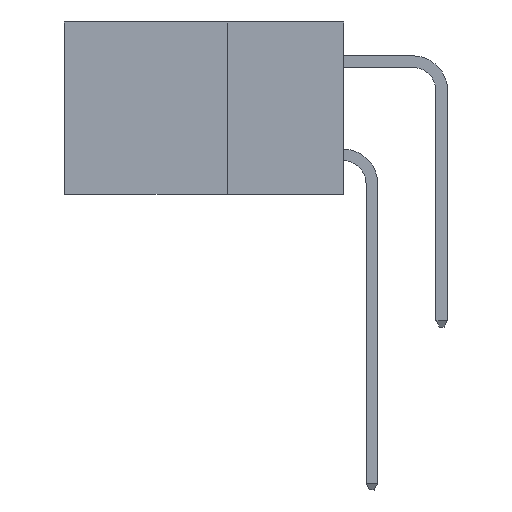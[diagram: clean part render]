
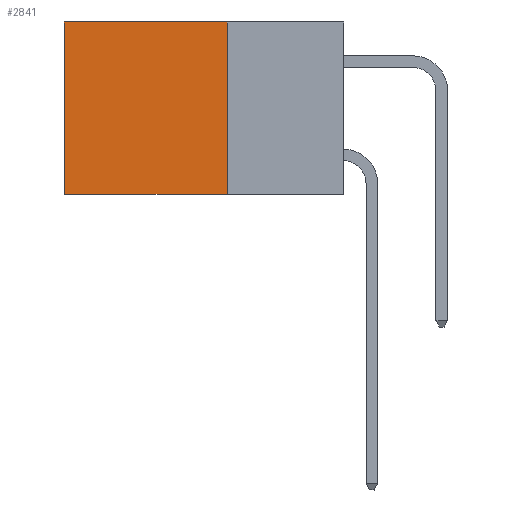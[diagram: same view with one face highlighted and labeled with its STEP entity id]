
A CAD part, left-side view. The second image highlights one B-rep face of the part: STEP entity #2841.
In plain terms, the highlighted planar face has unit normal (-1, 0, 0).
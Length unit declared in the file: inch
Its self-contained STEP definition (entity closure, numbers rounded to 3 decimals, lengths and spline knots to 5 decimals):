
#200 = CARTESIAN_POINT ( 'NONE',  ( 0.298, 0.25, -0.37 ) ) ;
#350 = EDGE_CURVE ( 'NONE', #2766, #12796, #1570, .T. ) ;
#964 = LINE ( 'NONE', #6120, #3939 ) ;
#1142 = VECTOR ( 'NONE', #9145, 39.37008 ) ;
#1369 = VECTOR ( 'NONE', #1447, 39.37008 ) ;
#1447 = DIRECTION ( 'NONE',  ( 0., 1., 0. ) ) ;
#1570 = LINE ( 'NONE', #13937, #1966 ) ;
#1756 = LINE ( 'NONE', #200, #1369 ) ;
#1966 = VECTOR ( 'NONE', #3776, 39.37008 ) ;
#2536 = DIRECTION ( 'NONE',  ( 0., 0., -1. ) ) ;
#2766 = VERTEX_POINT ( 'NONE', #13608 ) ;
#2841 = ADVANCED_FACE ( 'NONE', ( #4529 ), #12402, .F. ) ;
#2877 = CARTESIAN_POINT ( 'NONE',  ( 0.298, 0.25, 0. ) ) ;
#3033 = CARTESIAN_POINT ( 'NONE',  ( 0.298, 0.6, 0. ) ) ;
#3776 = DIRECTION ( 'NONE',  ( 0., 0., -1. ) ) ;
#3939 = VECTOR ( 'NONE', #9715, 39.37008 ) ;
#4529 = FACE_OUTER_BOUND ( 'NONE', #15367, .T. ) ;
#5228 = ORIENTED_EDGE ( 'NONE', *, *, #8145, .F. ) ;
#5418 = CARTESIAN_POINT ( 'NONE',  ( 0.298, 0.25, -0.37 ) ) ;
#5956 = ORIENTED_EDGE ( 'NONE', *, *, #8624, .T. ) ;
#5990 = AXIS2_PLACEMENT_3D ( 'NONE', #2877, #7428, #2536 ) ;
#6120 = CARTESIAN_POINT ( 'NONE',  ( 0.298, 0.25, 0. ) ) ;
#6282 = ORIENTED_EDGE ( 'NONE', *, *, #350, .F. ) ;
#6827 = ORIENTED_EDGE ( 'NONE', *, *, #13839, .T. ) ;
#7428 = DIRECTION ( 'NONE',  ( 1., 0., 0. ) ) ;
#7931 = CARTESIAN_POINT ( 'NONE',  ( 0.298, 0.6, -0.37 ) ) ;
#8145 = EDGE_CURVE ( 'NONE', #12796, #10522, #1756, .T. ) ;
#8202 = VERTEX_POINT ( 'NONE', #14853 ) ;
#8624 = EDGE_CURVE ( 'NONE', #2766, #8202, #964, .T. ) ;
#9145 = DIRECTION ( 'NONE',  ( 0., 0., -1. ) ) ;
#9715 = DIRECTION ( 'NONE',  ( 0., 1., 0. ) ) ;
#10522 = VERTEX_POINT ( 'NONE', #7931 ) ;
#11265 = LINE ( 'NONE', #3033, #1142 ) ;
#12402 = PLANE ( 'NONE',  #5990 ) ;
#12796 = VERTEX_POINT ( 'NONE', #5418 ) ;
#13608 = CARTESIAN_POINT ( 'NONE',  ( 0.298, 0.25, 0. ) ) ;
#13839 = EDGE_CURVE ( 'NONE', #8202, #10522, #11265, .T. ) ;
#13937 = CARTESIAN_POINT ( 'NONE',  ( 0.298, 0.25, 0. ) ) ;
#14853 = CARTESIAN_POINT ( 'NONE',  ( 0.298, 0.6, 0. ) ) ;
#15367 = EDGE_LOOP ( 'NONE', ( #6827, #5228, #6282, #5956 ) ) ;
